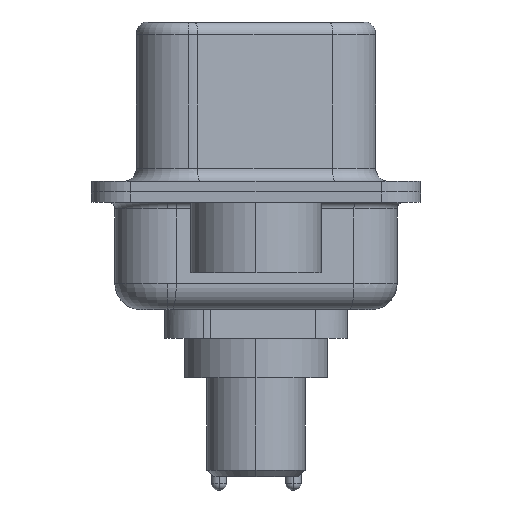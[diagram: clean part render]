
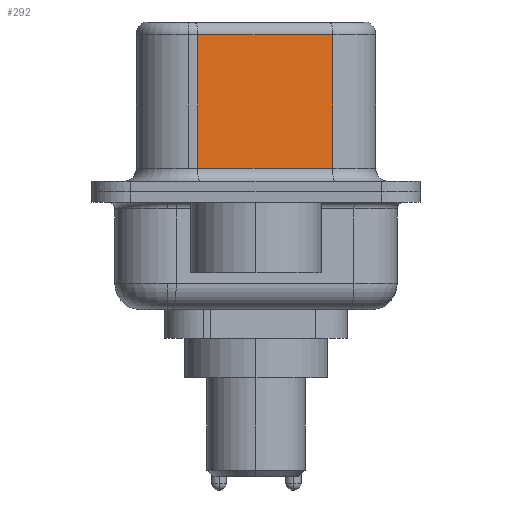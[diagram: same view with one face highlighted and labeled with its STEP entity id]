
A CAD part, left-side view. The second image highlights one B-rep face of the part: STEP entity #292.
In plain terms, the highlighted planar face has unit normal (-0.985, -0.174, 0).
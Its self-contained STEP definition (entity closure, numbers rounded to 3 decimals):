
#292 = ADVANCED_FACE ( 'NONE', ( #5890 ), #8397, .F. ) ;
#545 = CARTESIAN_POINT ( 'NONE',  ( 4.585, -2.927, 6.02 ) ) ;
#1256 = VECTOR ( 'NONE', #5842, 1000. ) ;
#1280 = EDGE_CURVE ( 'NONE', #7586, #5262, #9905, .T. ) ;
#1862 = VECTOR ( 'NONE', #15660, 1000. ) ;
#2538 = CARTESIAN_POINT ( 'NONE',  ( 3.675, 2.233, 0.9 ) ) ;
#3369 = ORIENTED_EDGE ( 'NONE', *, *, #5510, .T. ) ;
#3605 = EDGE_LOOP ( 'NONE', ( #8385, #5066, #3369, #14884 ) ) ;
#4096 = CARTESIAN_POINT ( 'NONE',  ( 4.585, -2.927, 6.02 ) ) ;
#4216 = LINE ( 'NONE', #11520, #7831 ) ;
#4341 = VERTEX_POINT ( 'NONE', #13166 ) ;
#5066 = ORIENTED_EDGE ( 'NONE', *, *, #14956, .T. ) ;
#5113 = DIRECTION ( 'NONE',  ( -0.174, 0.985, 0. ) ) ;
#5262 = VERTEX_POINT ( 'NONE', #15384 ) ;
#5466 = LINE ( 'NONE', #5652, #1862 ) ;
#5510 = EDGE_CURVE ( 'NONE', #4341, #11247, #5466, .T. ) ;
#5629 = VECTOR ( 'NONE', #13333, 1000. ) ;
#5652 = CARTESIAN_POINT ( 'NONE',  ( 3.675, 2.233, 6.52 ) ) ;
#5842 = DIRECTION ( 'NONE',  ( 0., 0., -1. ) ) ;
#5890 = FACE_OUTER_BOUND ( 'NONE', #3605, .T. ) ;
#6762 = DIRECTION ( 'NONE',  ( 0.985, 0.174, 0. ) ) ;
#7586 = VERTEX_POINT ( 'NONE', #545 ) ;
#7831 = VECTOR ( 'NONE', #13061, 1000. ) ;
#8385 = ORIENTED_EDGE ( 'NONE', *, *, #1280, .F. ) ;
#8397 = PLANE ( 'NONE',  #17488 ) ;
#9905 = LINE ( 'NONE', #17878, #1256 ) ;
#11247 = VERTEX_POINT ( 'NONE', #2538 ) ;
#11520 = CARTESIAN_POINT ( 'NONE',  ( 4.585, -2.927, 0.9 ) ) ;
#12290 = EDGE_CURVE ( 'NONE', #11247, #5262, #4216, .T. ) ;
#13061 = DIRECTION ( 'NONE',  ( 0.174, -0.985, 0. ) ) ;
#13166 = CARTESIAN_POINT ( 'NONE',  ( 3.675, 2.233, 6.02 ) ) ;
#13333 = DIRECTION ( 'NONE',  ( -0.174, 0.985, 0. ) ) ;
#14884 = ORIENTED_EDGE ( 'NONE', *, *, #12290, .T. ) ;
#14956 = EDGE_CURVE ( 'NONE', #7586, #4341, #17338, .T. ) ;
#15384 = CARTESIAN_POINT ( 'NONE',  ( 4.585, -2.927, 0.9 ) ) ;
#15660 = DIRECTION ( 'NONE',  ( 0., 0., -1. ) ) ;
#17338 = LINE ( 'NONE', #4096, #5629 ) ;
#17488 = AXIS2_PLACEMENT_3D ( 'NONE', #19856, #6762, #5113 ) ;
#17878 = CARTESIAN_POINT ( 'NONE',  ( 4.585, -2.927, 6.52 ) ) ;
#19856 = CARTESIAN_POINT ( 'NONE',  ( 4.585, -2.927, 6.52 ) ) ;
